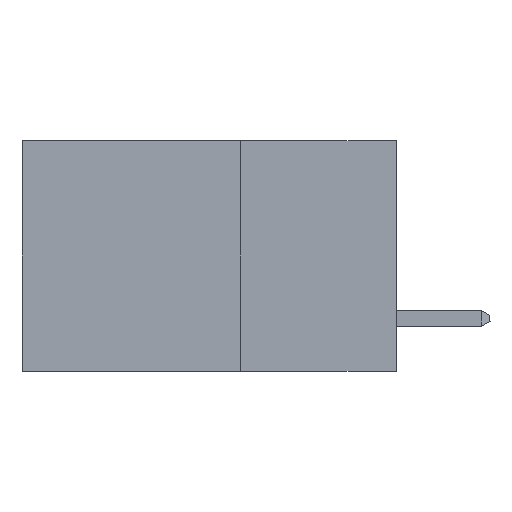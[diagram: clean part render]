
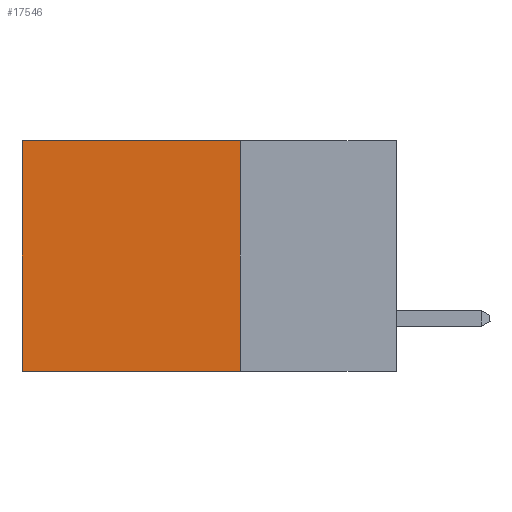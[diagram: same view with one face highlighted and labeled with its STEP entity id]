
A CAD part, left-side view. The second image highlights one B-rep face of the part: STEP entity #17546.
In plain terms, the highlighted planar face has unit normal (-1, 0, 0).
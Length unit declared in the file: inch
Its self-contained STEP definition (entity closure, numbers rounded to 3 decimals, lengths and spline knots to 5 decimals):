
#450 = EDGE_CURVE ( 'NONE', #16271, #15026, #7746, .T. ) ;
#892 = LINE ( 'NONE', #7446, #16939 ) ;
#1034 = VERTEX_POINT ( 'NONE', #2832 ) ;
#1448 = CARTESIAN_POINT ( 'NONE',  ( 0.298, 0.25, -0.37 ) ) ;
#2369 = CARTESIAN_POINT ( 'NONE',  ( 0.298, 0.25, 0. ) ) ;
#2832 = CARTESIAN_POINT ( 'NONE',  ( 0.298, 0.6, -0.37 ) ) ;
#3001 = CARTESIAN_POINT ( 'NONE',  ( 0.298, 0.6, 0. ) ) ;
#3770 = EDGE_CURVE ( 'NONE', #15026, #1034, #11385, .T. ) ;
#5698 = EDGE_CURVE ( 'NONE', #16271, #18827, #10563, .T. ) ;
#6184 = DIRECTION ( 'NONE',  ( 0., 0., -1. ) ) ;
#6316 = FACE_OUTER_BOUND ( 'NONE', #18007, .T. ) ;
#6889 = DIRECTION ( 'NONE',  ( 1., 0., 0. ) ) ;
#7001 = CARTESIAN_POINT ( 'NONE',  ( 0.298, 0.25, 0. ) ) ;
#7446 = CARTESIAN_POINT ( 'NONE',  ( 0.298, 0.25, -0.37 ) ) ;
#7746 = LINE ( 'NONE', #15353, #12240 ) ;
#8324 = DIRECTION ( 'NONE',  ( 0., 1., 0. ) ) ;
#9616 = VECTOR ( 'NONE', #6184, 39.37008 ) ;
#10389 = ORIENTED_EDGE ( 'NONE', *, *, #450, .T. ) ;
#10563 = LINE ( 'NONE', #12190, #9616 ) ;
#11385 = LINE ( 'NONE', #3001, #15386 ) ;
#11391 = EDGE_CURVE ( 'NONE', #18827, #1034, #892, .T. ) ;
#12007 = DIRECTION ( 'NONE',  ( 0., 1., 0. ) ) ;
#12190 = CARTESIAN_POINT ( 'NONE',  ( 0.298, 0.25, 0. ) ) ;
#12240 = VECTOR ( 'NONE', #8324, 39.37008 ) ;
#12379 = AXIS2_PLACEMENT_3D ( 'NONE', #2369, #6889, #17415 ) ;
#12897 = PLANE ( 'NONE',  #12379 ) ;
#13521 = DIRECTION ( 'NONE',  ( 0., 0., -1. ) ) ;
#15026 = VERTEX_POINT ( 'NONE', #15873 ) ;
#15146 = ORIENTED_EDGE ( 'NONE', *, *, #5698, .F. ) ;
#15353 = CARTESIAN_POINT ( 'NONE',  ( 0.298, 0.25, 0. ) ) ;
#15386 = VECTOR ( 'NONE', #13521, 39.37008 ) ;
#15873 = CARTESIAN_POINT ( 'NONE',  ( 0.298, 0.6, 0. ) ) ;
#16271 = VERTEX_POINT ( 'NONE', #7001 ) ;
#16723 = ORIENTED_EDGE ( 'NONE', *, *, #3770, .T. ) ;
#16939 = VECTOR ( 'NONE', #12007, 39.37008 ) ;
#17415 = DIRECTION ( 'NONE',  ( 0., 0., -1. ) ) ;
#17546 = ADVANCED_FACE ( 'NONE', ( #6316 ), #12897, .F. ) ;
#18007 = EDGE_LOOP ( 'NONE', ( #16723, #19175, #15146, #10389 ) ) ;
#18827 = VERTEX_POINT ( 'NONE', #1448 ) ;
#19175 = ORIENTED_EDGE ( 'NONE', *, *, #11391, .F. ) ;
